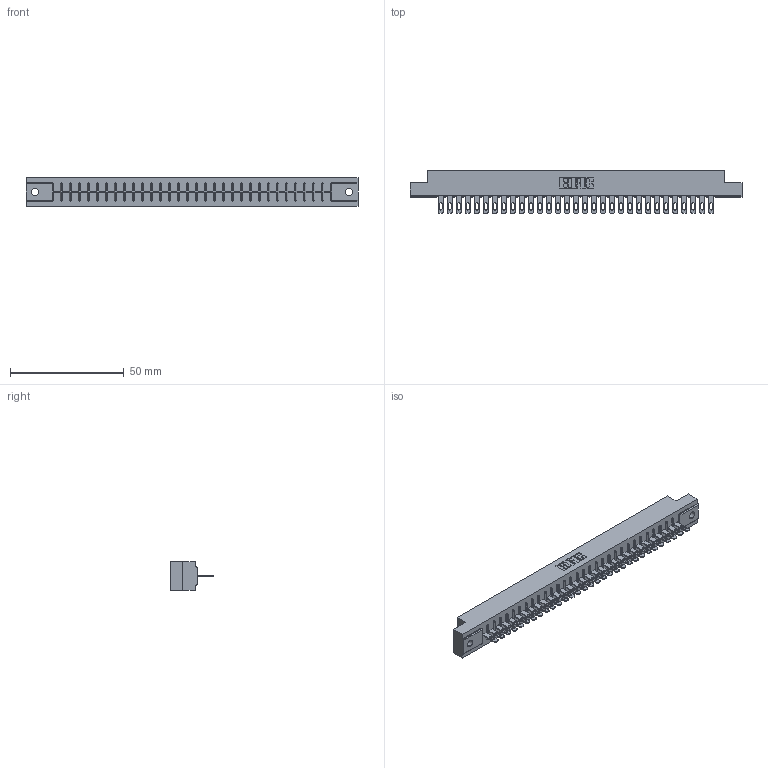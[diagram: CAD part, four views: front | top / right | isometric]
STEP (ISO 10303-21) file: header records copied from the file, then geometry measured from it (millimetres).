
FILE_DESCRIPTION (( 'STEP AP203' ), '1' );
FILE_NAME ('306-031-400-102.STEP', '2020-09-22T01:30:21', ( '' ), ( '' ), 'SwSTEP 2.0', 'SolidWorks 2020', '' );
FILE_SCHEMA (( 'CONFIG_CONTROL_DESIGN' ));
Length unit declared in the file: inch
Products named in the file (3): 306-031-400-102; 306 Part_.128 Dia; 306-290-001_100
Assembly tree (32 placements, depth 2):
  306-031-400-102
    306 Part_.128 Dia
    306-290-001_100  x31
Bounding box: 145.85 x 18.87 x 12.7 mm (x, y, z)
Volume: 16089.1 mm3; surface area: 16668.6 mm2
Topology: 32 solids, 32 shells, 2472 faces, 6981 edges, 4486 vertices
Faces by surface type: plane 1618, cylinder 730, sphere 124
Entity records: 30500 total; most frequent: CARTESIAN_POINT 5120, ORIENTED_EDGE 5074, DIRECTION 5051, EDGE_CURVE 2537, LINE 1977, VECTOR 1977, VERTEX_POINT 1606, AXIS2_PLACEMENT_3D 1537
